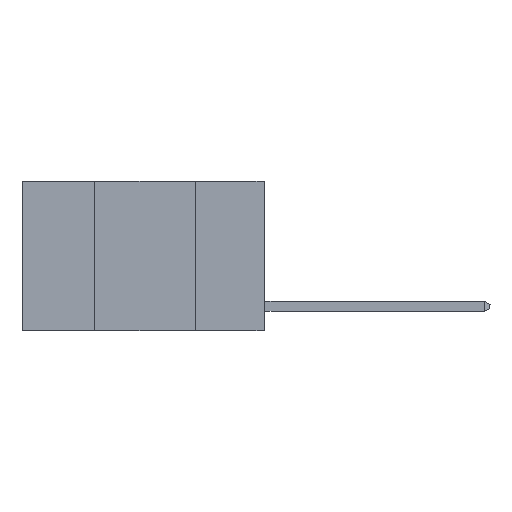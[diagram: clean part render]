
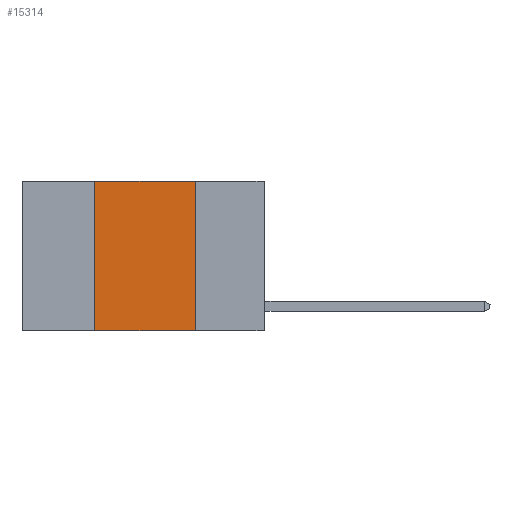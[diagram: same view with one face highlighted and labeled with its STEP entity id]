
A CAD part, left-side view. The second image highlights one B-rep face of the part: STEP entity #15314.
In plain terms, the highlighted planar face has unit normal (-1, 0, 0).
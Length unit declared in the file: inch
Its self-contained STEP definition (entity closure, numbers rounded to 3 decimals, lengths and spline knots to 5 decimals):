
#263 = DIRECTION ( 'NONE',  ( 0., -1., 0. ) ) ;
#420 = ORIENTED_EDGE ( 'NONE', *, *, #12475, .F. ) ;
#593 = VECTOR ( 'NONE', #2713, 39.37008 ) ;
#1196 = LINE ( 'NONE', #10598, #4048 ) ;
#1931 = LINE ( 'NONE', #7668, #593 ) ;
#2668 = EDGE_CURVE ( 'NONE', #7227, #5960, #1931, .T. ) ;
#2713 = DIRECTION ( 'NONE',  ( 0., 0., -1. ) ) ;
#2900 = ORIENTED_EDGE ( 'NONE', *, *, #2668, .F. ) ;
#2935 = LINE ( 'NONE', #6176, #3895 ) ;
#3895 = VECTOR ( 'NONE', #9870, 39.37008 ) ;
#3937 = AXIS2_PLACEMENT_3D ( 'NONE', #4647, #5896, #7273 ) ;
#4048 = VECTOR ( 'NONE', #14306, 39.37008 ) ;
#4120 = VECTOR ( 'NONE', #263, 39.37008 ) ;
#4568 = EDGE_CURVE ( 'NONE', #14608, #5960, #12339, .T. ) ;
#4647 = CARTESIAN_POINT ( 'NONE',  ( 0., 0.6, 0. ) ) ;
#4736 = VERTEX_POINT ( 'NONE', #12987 ) ;
#5896 = DIRECTION ( 'NONE',  ( 1., 0., 0. ) ) ;
#5960 = VERTEX_POINT ( 'NONE', #11208 ) ;
#5972 = CARTESIAN_POINT ( 'NONE',  ( 0., 0.17, 0. ) ) ;
#6176 = CARTESIAN_POINT ( 'NONE',  ( 0., 0.6, 0. ) ) ;
#7227 = VERTEX_POINT ( 'NONE', #5972 ) ;
#7273 = DIRECTION ( 'NONE',  ( 0., 0., -1. ) ) ;
#7565 = CARTESIAN_POINT ( 'NONE',  ( 0., 0.42, -0.37 ) ) ;
#7668 = CARTESIAN_POINT ( 'NONE',  ( 0., 0.17, 0. ) ) ;
#9870 = DIRECTION ( 'NONE',  ( 0., -1., 0. ) ) ;
#10598 = CARTESIAN_POINT ( 'NONE',  ( 0., 0.42, 0. ) ) ;
#11208 = CARTESIAN_POINT ( 'NONE',  ( 0., 0.17, -0.37 ) ) ;
#11401 = ORIENTED_EDGE ( 'NONE', *, *, #14555, .F. ) ;
#12339 = LINE ( 'NONE', #12720, #4120 ) ;
#12422 = FACE_OUTER_BOUND ( 'NONE', #12938, .T. ) ;
#12475 = EDGE_CURVE ( 'NONE', #4736, #7227, #2935, .T. ) ;
#12720 = CARTESIAN_POINT ( 'NONE',  ( 0., 0.6, -0.37 ) ) ;
#12938 = EDGE_LOOP ( 'NONE', ( #2900, #420, #11401, #14159 ) ) ;
#12987 = CARTESIAN_POINT ( 'NONE',  ( 0., 0.42, 0. ) ) ;
#14159 = ORIENTED_EDGE ( 'NONE', *, *, #4568, .T. ) ;
#14306 = DIRECTION ( 'NONE',  ( 0., 0., 1. ) ) ;
#14555 = EDGE_CURVE ( 'NONE', #14608, #4736, #1196, .T. ) ;
#14608 = VERTEX_POINT ( 'NONE', #7565 ) ;
#15314 = ADVANCED_FACE ( 'NONE', ( #12422 ), #15978, .F. ) ;
#15978 = PLANE ( 'NONE',  #3937 ) ;
